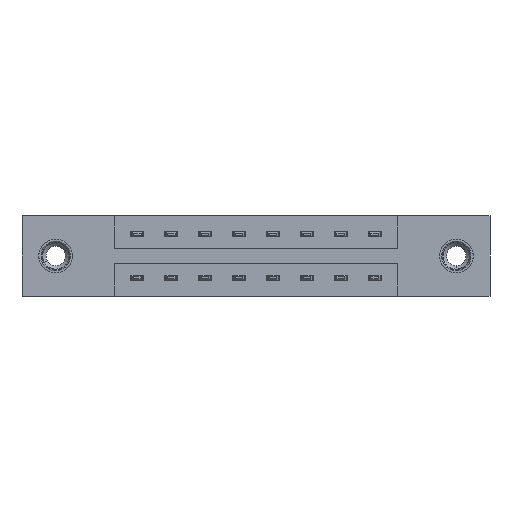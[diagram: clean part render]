
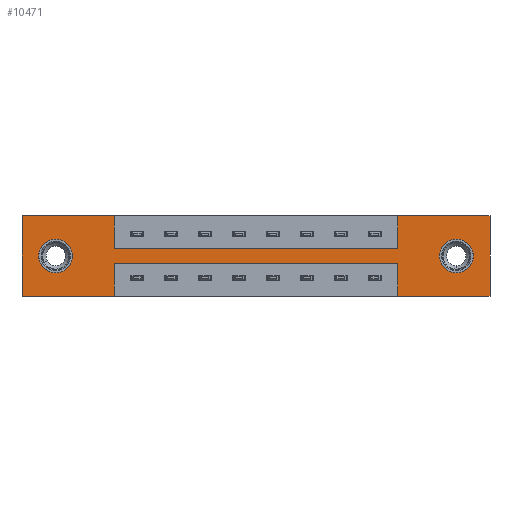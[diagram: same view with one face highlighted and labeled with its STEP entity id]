
A CAD part, front view. The second image highlights one B-rep face of the part: STEP entity #10471.
In plain terms, the highlighted planar face has unit normal (0, -1, 0).
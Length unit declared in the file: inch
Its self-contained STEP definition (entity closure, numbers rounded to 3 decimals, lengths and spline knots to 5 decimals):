
#78 = ORIENTED_EDGE ( 'NONE', *, *, #5109, .F. ) ;
#151 = EDGE_CURVE ( 'NONE', #11377, #1295, #9618, .T. ) ;
#193 = DIRECTION ( 'NONE',  ( 1., 0., 0. ) ) ;
#253 = EDGE_CURVE ( 'NONE', #1295, #1050, #10254, .T. ) ;
#328 = CARTESIAN_POINT ( 'NONE',  ( 1.729, 0., -0.15 ) ) ;
#405 = ORIENTED_EDGE ( 'NONE', *, *, #489, .F. ) ;
#413 = EDGE_CURVE ( 'NONE', #6716, #7781, #10514, .T. ) ;
#485 = EDGE_CURVE ( 'NONE', #8782, #6716, #3810, .T. ) ;
#489 = EDGE_CURVE ( 'NONE', #7781, #2575, #6244, .T. ) ;
#573 = ORIENTED_EDGE ( 'NONE', *, *, #413, .F. ) ;
#610 = DIRECTION ( 'NONE',  ( 1., 0., 0. ) ) ;
#736 = VERTEX_POINT ( 'NONE', #328 ) ;
#984 = VERTEX_POINT ( 'NONE', #5953 ) ;
#1050 = VERTEX_POINT ( 'NONE', #3919 ) ;
#1084 = DIRECTION ( 'NONE',  ( 0., 0., -1. ) ) ;
#1117 = EDGE_CURVE ( 'NONE', #5753, #8068, #3378, .T. ) ;
#1266 = VERTEX_POINT ( 'NONE', #5176 ) ;
#1295 = VERTEX_POINT ( 'NONE', #2446 ) ;
#1407 = VECTOR ( 'NONE', #2875, 39.37008 ) ;
#1412 = CARTESIAN_POINT ( 'NONE',  ( 1.729, 0., -0.37 ) ) ;
#1435 = DIRECTION ( 'NONE',  ( 0., 0., -1. ) ) ;
#1520 = DIRECTION ( 'NONE',  ( 0., 1., 0. ) ) ;
#1578 = CARTESIAN_POINT ( 'NONE',  ( 1.999, 0., -0.185 ) ) ;
#1879 = DIRECTION ( 'NONE',  ( 0., 1., 0. ) ) ;
#2040 = ORIENTED_EDGE ( 'NONE', *, *, #151, .F. ) ;
#2114 = VECTOR ( 'NONE', #10256, 39.37008 ) ;
#2135 = LINE ( 'NONE', #8483, #5058 ) ;
#2141 = DIRECTION ( 'NONE',  ( 1., 0., 0. ) ) ;
#2149 = EDGE_CURVE ( 'NONE', #7420, #9992, #10998, .T. ) ;
#2219 = DIRECTION ( 'NONE',  ( 0., 1., 0. ) ) ;
#2288 = AXIS2_PLACEMENT_3D ( 'NONE', #8869, #8806, #4990 ) ;
#2303 = CARTESIAN_POINT ( 'NONE',  ( 2.154, 0., 0. ) ) ;
#2446 = CARTESIAN_POINT ( 'NONE',  ( 2.154, 0., -0.37 ) ) ;
#2452 = VECTOR ( 'NONE', #8071, 39.37008 ) ;
#2575 = VERTEX_POINT ( 'NONE', #7163 ) ;
#2657 = AXIS2_PLACEMENT_3D ( 'NONE', #11300, #11343, #6116 ) ;
#2658 = EDGE_CURVE ( 'NONE', #736, #3188, #8764, .T. ) ;
#2795 = CARTESIAN_POINT ( 'NONE',  ( 0.155, 0., -0.263 ) ) ;
#2828 = CARTESIAN_POINT ( 'NONE',  ( 1.999, 0., -0.263 ) ) ;
#2875 = DIRECTION ( 'NONE',  ( -1., 0., 0. ) ) ;
#2958 = LINE ( 'NONE', #4746, #9554 ) ;
#2981 = AXIS2_PLACEMENT_3D ( 'NONE', #4144, #2219, #1084 ) ;
#3042 = CARTESIAN_POINT ( 'NONE',  ( 1.729, 0., -0.22 ) ) ;
#3075 = CARTESIAN_POINT ( 'NONE',  ( 0., 0., -0.37 ) ) ;
#3085 = CARTESIAN_POINT ( 'NONE',  ( 0.425, 0., 0. ) ) ;
#3156 = EDGE_CURVE ( 'NONE', #8068, #5753, #10457, .T. ) ;
#3188 = VERTEX_POINT ( 'NONE', #6962 ) ;
#3295 = ORIENTED_EDGE ( 'NONE', *, *, #9634, .F. ) ;
#3378 = CIRCLE ( 'NONE', #3538, 0.078 ) ;
#3409 = CARTESIAN_POINT ( 'NONE',  ( 0., 0., 0. ) ) ;
#3534 = DIRECTION ( 'NONE',  ( 0., 0., -1. ) ) ;
#3538 = AXIS2_PLACEMENT_3D ( 'NONE', #1578, #1520, #1435 ) ;
#3678 = VECTOR ( 'NONE', #3534, 39.37008 ) ;
#3810 = LINE ( 'NONE', #7200, #1407 ) ;
#3919 = CARTESIAN_POINT ( 'NONE',  ( 1.729, 0., -0.37 ) ) ;
#3988 = ORIENTED_EDGE ( 'NONE', *, *, #3156, .T. ) ;
#4081 = VECTOR ( 'NONE', #9958, 39.37008 ) ;
#4144 = CARTESIAN_POINT ( 'NONE',  ( 1.999, 0., -0.185 ) ) ;
#4219 = CARTESIAN_POINT ( 'NONE',  ( 1.729, 0., 0. ) ) ;
#4247 = EDGE_CURVE ( 'NONE', #3188, #11377, #7038, .T. ) ;
#4269 = AXIS2_PLACEMENT_3D ( 'NONE', #7322, #1879, #8226 ) ;
#4416 = EDGE_CURVE ( 'NONE', #1266, #736, #2135, .T. ) ;
#4607 = LINE ( 'NONE', #8435, #9176 ) ;
#4665 = ORIENTED_EDGE ( 'NONE', *, *, #4416, .F. ) ;
#4746 = CARTESIAN_POINT ( 'NONE',  ( 0., 0., 0. ) ) ;
#4938 = FACE_OUTER_BOUND ( 'NONE', #9308, .T. ) ;
#4959 = ORIENTED_EDGE ( 'NONE', *, *, #7352, .F. ) ;
#4990 = DIRECTION ( 'NONE',  ( 0., 0., 1. ) ) ;
#5058 = VECTOR ( 'NONE', #2141, 39.37008 ) ;
#5109 = EDGE_CURVE ( 'NONE', #8268, #1266, #4607, .T. ) ;
#5175 = PLANE ( 'NONE',  #2657 ) ;
#5176 = CARTESIAN_POINT ( 'NONE',  ( 0.425, 0., -0.15 ) ) ;
#5230 = VECTOR ( 'NONE', #6202, 39.37008 ) ;
#5603 = CARTESIAN_POINT ( 'NONE',  ( 1.999, 0., -0.107 ) ) ;
#5640 = DIRECTION ( 'NONE',  ( 0., 0., 1. ) ) ;
#5753 = VERTEX_POINT ( 'NONE', #5603 ) ;
#5805 = EDGE_CURVE ( 'NONE', #2575, #984, #2958, .T. ) ;
#5953 = CARTESIAN_POINT ( 'NONE',  ( 0., 0., 0. ) ) ;
#6038 = CARTESIAN_POINT ( 'NONE',  ( 2.154, 0., 0. ) ) ;
#6061 = CARTESIAN_POINT ( 'NONE',  ( 0., 0., 0. ) ) ;
#6116 = DIRECTION ( 'NONE',  ( 0., 0., -1. ) ) ;
#6202 = DIRECTION ( 'NONE',  ( -1., 0., 0. ) ) ;
#6244 = LINE ( 'NONE', #10607, #4081 ) ;
#6273 = LINE ( 'NONE', #1412, #8693 ) ;
#6645 = EDGE_LOOP ( 'NONE', ( #9381, #9638 ) ) ;
#6716 = VERTEX_POINT ( 'NONE', #10352 ) ;
#6717 = EDGE_LOOP ( 'NONE', ( #10797, #3988 ) ) ;
#6863 = ORIENTED_EDGE ( 'NONE', *, *, #4247, .F. ) ;
#6962 = CARTESIAN_POINT ( 'NONE',  ( 1.729, 0., 0. ) ) ;
#6987 = CARTESIAN_POINT ( 'NONE',  ( 0.425, 0., -0.37 ) ) ;
#7038 = LINE ( 'NONE', #3409, #9400 ) ;
#7163 = CARTESIAN_POINT ( 'NONE',  ( 0., 0., -0.37 ) ) ;
#7200 = CARTESIAN_POINT ( 'NONE',  ( 0.425, 0., -0.22 ) ) ;
#7319 = CARTESIAN_POINT ( 'NONE',  ( 0.425, 0., -0.37 ) ) ;
#7322 = CARTESIAN_POINT ( 'NONE',  ( 0.155, 0., -0.185 ) ) ;
#7352 = EDGE_CURVE ( 'NONE', #984, #8268, #10450, .T. ) ;
#7420 = VERTEX_POINT ( 'NONE', #10532 ) ;
#7454 = ORIENTED_EDGE ( 'NONE', *, *, #5805, .F. ) ;
#7591 = ORIENTED_EDGE ( 'NONE', *, *, #485, .F. ) ;
#7716 = FACE_BOUND ( 'NONE', #6645, .T. ) ;
#7723 = CIRCLE ( 'NONE', #4269, 0.078 ) ;
#7781 = VERTEX_POINT ( 'NONE', #6987 ) ;
#7800 = DIRECTION ( 'NONE',  ( 0., 0., 1. ) ) ;
#8068 = VERTEX_POINT ( 'NONE', #2828 ) ;
#8071 = DIRECTION ( 'NONE',  ( 0., 0., -1. ) ) ;
#8226 = DIRECTION ( 'NONE',  ( 0., 0., 1. ) ) ;
#8268 = VERTEX_POINT ( 'NONE', #3085 ) ;
#8435 = CARTESIAN_POINT ( 'NONE',  ( 0.425, 0., 0. ) ) ;
#8483 = CARTESIAN_POINT ( 'NONE',  ( 0.425, 0., -0.15 ) ) ;
#8693 = VECTOR ( 'NONE', #7800, 39.37008 ) ;
#8764 = LINE ( 'NONE', #4219, #2114 ) ;
#8782 = VERTEX_POINT ( 'NONE', #3042 ) ;
#8806 = DIRECTION ( 'NONE',  ( 0., 1., 0. ) ) ;
#8869 = CARTESIAN_POINT ( 'NONE',  ( 0.155, 0., -0.185 ) ) ;
#8966 = ORIENTED_EDGE ( 'NONE', *, *, #253, .F. ) ;
#9176 = VECTOR ( 'NONE', #9295, 39.37008 ) ;
#9233 = ORIENTED_EDGE ( 'NONE', *, *, #2658, .F. ) ;
#9295 = DIRECTION ( 'NONE',  ( 0., 0., -1. ) ) ;
#9308 = EDGE_LOOP ( 'NONE', ( #573, #7591, #3295, #8966, #2040, #6863, #9233, #4665, #78, #4959, #7454, #405 ) ) ;
#9381 = ORIENTED_EDGE ( 'NONE', *, *, #2149, .T. ) ;
#9400 = VECTOR ( 'NONE', #193, 39.37008 ) ;
#9476 = FACE_BOUND ( 'NONE', #6717, .T. ) ;
#9554 = VECTOR ( 'NONE', #5640, 39.37008 ) ;
#9618 = LINE ( 'NONE', #6038, #2452 ) ;
#9634 = EDGE_CURVE ( 'NONE', #1050, #8782, #6273, .T. ) ;
#9638 = ORIENTED_EDGE ( 'NONE', *, *, #9969, .T. ) ;
#9958 = DIRECTION ( 'NONE',  ( -1., 0., 0. ) ) ;
#9969 = EDGE_CURVE ( 'NONE', #9992, #7420, #7723, .T. ) ;
#9992 = VERTEX_POINT ( 'NONE', #2795 ) ;
#10254 = LINE ( 'NONE', #3075, #5230 ) ;
#10256 = DIRECTION ( 'NONE',  ( 0., 0., 1. ) ) ;
#10352 = CARTESIAN_POINT ( 'NONE',  ( 0.425, 0., -0.22 ) ) ;
#10450 = LINE ( 'NONE', #6061, #10969 ) ;
#10457 = CIRCLE ( 'NONE', #2981, 0.078 ) ;
#10471 = ADVANCED_FACE ( 'NONE', ( #9476, #7716, #4938 ), #5175, .T. ) ;
#10514 = LINE ( 'NONE', #7319, #3678 ) ;
#10532 = CARTESIAN_POINT ( 'NONE',  ( 0.155, 0., -0.107 ) ) ;
#10607 = CARTESIAN_POINT ( 'NONE',  ( 0., 0., -0.37 ) ) ;
#10797 = ORIENTED_EDGE ( 'NONE', *, *, #1117, .T. ) ;
#10969 = VECTOR ( 'NONE', #610, 39.37008 ) ;
#10998 = CIRCLE ( 'NONE', #2288, 0.078 ) ;
#11300 = CARTESIAN_POINT ( 'NONE',  ( 0., 0., -0.37 ) ) ;
#11343 = DIRECTION ( 'NONE',  ( 0., -1., 0. ) ) ;
#11377 = VERTEX_POINT ( 'NONE', #2303 ) ;
